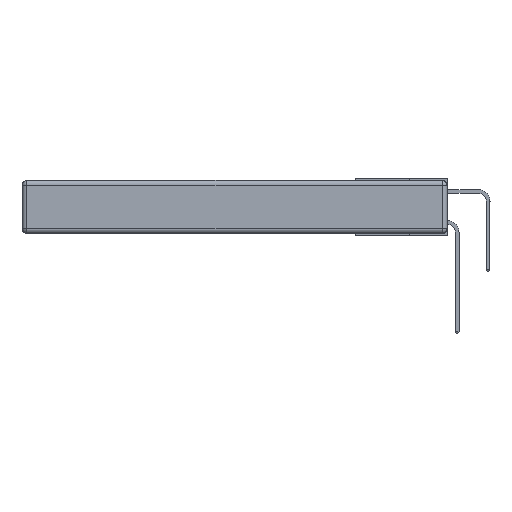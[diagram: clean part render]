
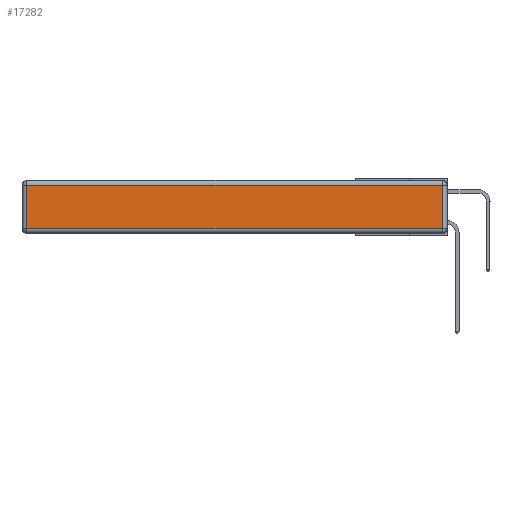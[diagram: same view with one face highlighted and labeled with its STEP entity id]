
A CAD part, left-side view. The second image highlights one B-rep face of the part: STEP entity #17282.
In plain terms, the highlighted planar face has unit normal (-1, 0, 0).
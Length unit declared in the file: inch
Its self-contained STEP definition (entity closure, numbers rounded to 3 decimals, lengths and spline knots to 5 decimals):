
#1377 = VERTEX_POINT ( 'NONE', #18963 ) ;
#2318 = VERTEX_POINT ( 'NONE', #27978 ) ;
#2881 = CARTESIAN_POINT ( 'NONE',  ( 0., 2.72, -0.343 ) ) ;
#2963 = ORIENTED_EDGE ( 'NONE', *, *, #28388, .T. ) ;
#3978 = DIRECTION ( 'NONE',  ( 0., 0., 1. ) ) ;
#4088 = CARTESIAN_POINT ( 'NONE',  ( 0., 0., -0.343 ) ) ;
#4624 = CARTESIAN_POINT ( 'NONE',  ( 0., 0.03, -0.03 ) ) ;
#5332 = EDGE_CURVE ( 'NONE', #2318, #23829, #21440, .T. ) ;
#6468 = FACE_OUTER_BOUND ( 'NONE', #19996, .T. ) ;
#6866 = VECTOR ( 'NONE', #7198, 39.37008 ) ;
#7173 = VECTOR ( 'NONE', #24650, 39.37008 ) ;
#7198 = DIRECTION ( 'NONE',  ( 0., 1., 0. ) ) ;
#7811 = AXIS2_PLACEMENT_3D ( 'NONE', #4088, #10835, #3978 ) ;
#9044 = LINE ( 'NONE', #2881, #19953 ) ;
#10835 = DIRECTION ( 'NONE',  ( -1., 0., 0. ) ) ;
#12751 = CARTESIAN_POINT ( 'NONE',  ( 0., 0., -0.313 ) ) ;
#13785 = ORIENTED_EDGE ( 'NONE', *, *, #5332, .T. ) ;
#15006 = DIRECTION ( 'NONE',  ( 0., -1., 0. ) ) ;
#16156 = VERTEX_POINT ( 'NONE', #4624 ) ;
#17282 = ADVANCED_FACE ( 'NONE', ( #6468 ), #17867, .T. ) ;
#17683 = LINE ( 'NONE', #29349, #7173 ) ;
#17867 = PLANE ( 'NONE',  #7811 ) ;
#18866 = CARTESIAN_POINT ( 'NONE',  ( 0., 2.75, -0.03 ) ) ;
#18963 = CARTESIAN_POINT ( 'NONE',  ( 0., 2.72, -0.03 ) ) ;
#19953 = VECTOR ( 'NONE', #21506, 39.37008 ) ;
#19996 = EDGE_LOOP ( 'NONE', ( #13785, #2963, #26700, #25691 ) ) ;
#21440 = LINE ( 'NONE', #12751, #29086 ) ;
#21506 = DIRECTION ( 'NONE',  ( 0., 0., -1. ) ) ;
#21768 = CARTESIAN_POINT ( 'NONE',  ( 0., 0.03, -0.313 ) ) ;
#22266 = EDGE_CURVE ( 'NONE', #16156, #1377, #25024, .T. ) ;
#23829 = VERTEX_POINT ( 'NONE', #21768 ) ;
#24650 = DIRECTION ( 'NONE',  ( 0., 0., 1. ) ) ;
#25024 = LINE ( 'NONE', #18866, #6866 ) ;
#25691 = ORIENTED_EDGE ( 'NONE', *, *, #27702, .T. ) ;
#26700 = ORIENTED_EDGE ( 'NONE', *, *, #22266, .T. ) ;
#27702 = EDGE_CURVE ( 'NONE', #1377, #2318, #9044, .T. ) ;
#27978 = CARTESIAN_POINT ( 'NONE',  ( 0., 2.72, -0.313 ) ) ;
#28388 = EDGE_CURVE ( 'NONE', #23829, #16156, #17683, .T. ) ;
#29086 = VECTOR ( 'NONE', #15006, 39.37008 ) ;
#29349 = CARTESIAN_POINT ( 'NONE',  ( 0., 0.03, -0.343 ) ) ;
